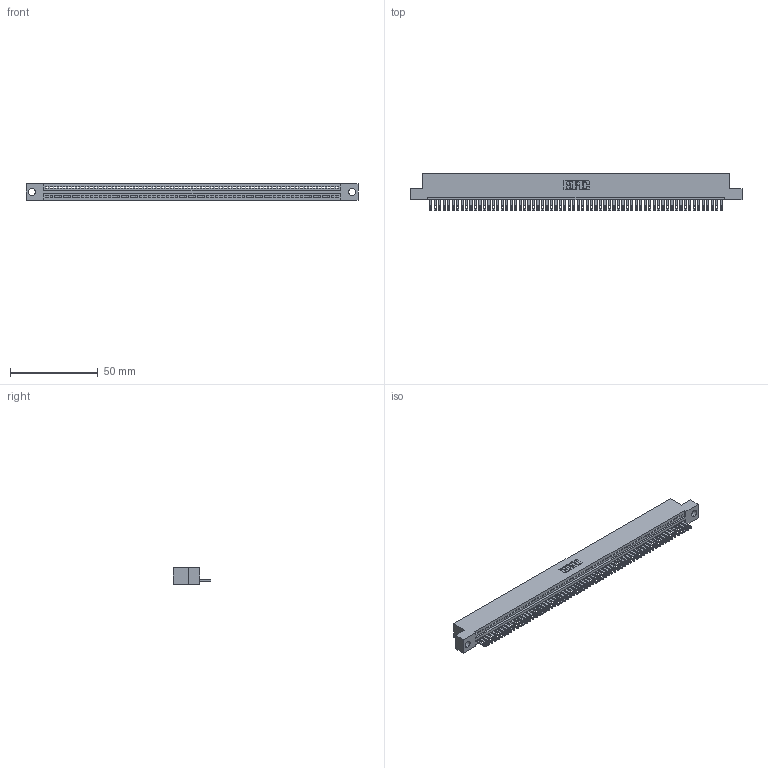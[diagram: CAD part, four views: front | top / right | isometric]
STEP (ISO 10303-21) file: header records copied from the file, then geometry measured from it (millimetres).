
FILE_DESCRIPTION (( 'STEP AP203' ), '1' );
FILE_NAME ('895-066-500-104.STEP', '2020-09-28T12:04:56', ( '' ), ( '' ), 'SwSTEP 2.0', 'SolidWorks 2020', '' );
FILE_SCHEMA (( 'CONFIG_CONTROL_DESIGN' ));
Length unit declared in the file: inch
Products named in the file (3): 845 Part_Flush Mounting Lugs - 0.156 Dia-TH; 895-066-500-104; 345-292-001_345-293-100
Assembly tree (67 placements, depth 2):
  895-066-500-104
    845 Part_Flush Mounting Lugs - 0.156 Dia-TH
    345-292-001_345-293-100  x66
Bounding box: 188.85 x 21.51 x 9.4 mm (x, y, z)
Volume: 18086.7 mm3; surface area: 24318.7 mm2
Topology: 67 solids, 67 shells, 3690 faces, 11429 edges, 7618 vertices
Faces by surface type: plane 2324, cylinder 1366
Entity records: 46375 total; most frequent: ORIENTED_EDGE 8038, CARTESIAN_POINT 8038, DIRECTION 6987, EDGE_CURVE 4019, LINE 3619, VECTOR 3619, VERTEX_POINT 2678, AXIS2_PLACEMENT_3D 1684
